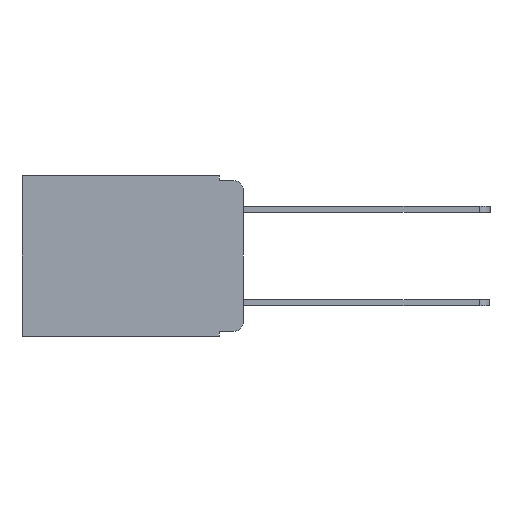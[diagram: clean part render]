
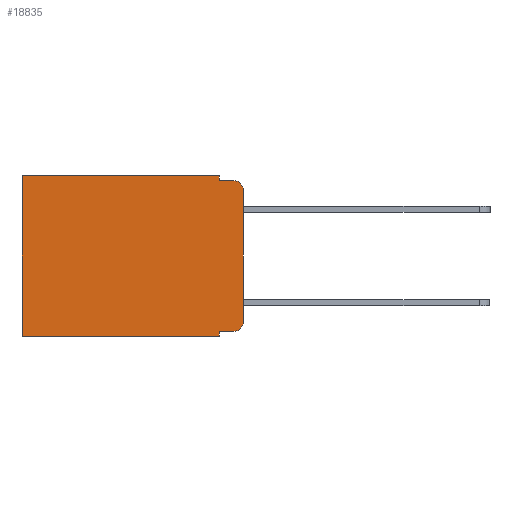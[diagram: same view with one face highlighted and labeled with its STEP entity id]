
A CAD part, left-side view. The second image highlights one B-rep face of the part: STEP entity #18835.
In plain terms, the highlighted planar face has unit normal (-1, 0, 0).
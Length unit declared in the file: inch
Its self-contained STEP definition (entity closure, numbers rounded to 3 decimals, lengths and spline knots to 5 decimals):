
#89 = VERTEX_POINT ( 'NONE', #7108 ) ;
#629 = ORIENTED_EDGE ( 'NONE', *, *, #4387, .T. ) ;
#857 = VERTEX_POINT ( 'NONE', #22452 ) ;
#1180 = FACE_OUTER_BOUND ( 'NONE', #19927, .T. ) ;
#1786 = CARTESIAN_POINT ( 'NONE',  ( 0.298, 0.051, -0.343 ) ) ;
#1888 = CARTESIAN_POINT ( 'NONE',  ( 0.298, 0.02, -0.03 ) ) ;
#2769 = CARTESIAN_POINT ( 'NONE',  ( 0.298, 0., 0. ) ) ;
#2882 = CARTESIAN_POINT ( 'NONE',  ( 0.298, 0., -0.03 ) ) ;
#2957 = CARTESIAN_POINT ( 'NONE',  ( 0.298, 0.051, -0.01 ) ) ;
#3041 = VERTEX_POINT ( 'NONE', #2882 ) ;
#3230 = VERTEX_POINT ( 'NONE', #14406 ) ;
#3738 = DIRECTION ( 'NONE',  ( 0., 0., -1. ) ) ;
#4284 = LINE ( 'NONE', #2769, #21764 ) ;
#4387 = EDGE_CURVE ( 'NONE', #3041, #89, #19118, .T. ) ;
#4490 = EDGE_CURVE ( 'NONE', #5047, #8650, #21510, .T. ) ;
#4580 = VERTEX_POINT ( 'NONE', #14867 ) ;
#4734 = EDGE_CURVE ( 'NONE', #3041, #9406, #4284, .T. ) ;
#4835 = CARTESIAN_POINT ( 'NONE',  ( 0.298, 0.051, -0.333 ) ) ;
#5047 = VERTEX_POINT ( 'NONE', #1786 ) ;
#5217 = AXIS2_PLACEMENT_3D ( 'NONE', #8391, #20550, #10196 ) ;
#5502 = EDGE_CURVE ( 'NONE', #4580, #18981, #6504, .T. ) ;
#5528 = VECTOR ( 'NONE', #20589, 39.37008 ) ;
#5563 = LINE ( 'NONE', #18065, #11428 ) ;
#5821 = DIRECTION ( 'NONE',  ( 0., 0., -1. ) ) ;
#6057 = CARTESIAN_POINT ( 'NONE',  ( 0.298, 0., 0. ) ) ;
#6140 = DIRECTION ( 'NONE',  ( 0., 0., -1. ) ) ;
#6504 = LINE ( 'NONE', #6858, #19861 ) ;
#6658 = ORIENTED_EDGE ( 'NONE', *, *, #5502, .F. ) ;
#6824 = CARTESIAN_POINT ( 'NONE',  ( 0.298, 0., -0.313 ) ) ;
#6858 = CARTESIAN_POINT ( 'NONE',  ( 0.298, 0.051, 0. ) ) ;
#7108 = CARTESIAN_POINT ( 'NONE',  ( 0.298, 0.02, -0.01 ) ) ;
#7143 = DIRECTION ( 'NONE',  ( 0., 1., 0. ) ) ;
#7154 = EDGE_CURVE ( 'NONE', #12193, #8650, #5563, .T. ) ;
#7475 = EDGE_CURVE ( 'NONE', #4580, #12193, #20570, .T. ) ;
#7652 = VECTOR ( 'NONE', #21484, 39.37008 ) ;
#7845 = DIRECTION ( 'NONE',  ( 1., 0., 0. ) ) ;
#7990 = EDGE_CURVE ( 'NONE', #18981, #89, #19481, .T. ) ;
#8359 = ORIENTED_EDGE ( 'NONE', *, *, #17285, .T. ) ;
#8391 = CARTESIAN_POINT ( 'NONE',  ( 0.298, 0.02, -0.313 ) ) ;
#8650 = VERTEX_POINT ( 'NONE', #13787 ) ;
#9406 = VERTEX_POINT ( 'NONE', #6824 ) ;
#9649 = VECTOR ( 'NONE', #6140, 39.37008 ) ;
#10167 = AXIS2_PLACEMENT_3D ( 'NONE', #6057, #7845, #20012 ) ;
#10196 = DIRECTION ( 'NONE',  ( 0., 0., -1. ) ) ;
#10237 = CARTESIAN_POINT ( 'NONE',  ( 0.298, 0.051, -0.01 ) ) ;
#10572 = ORIENTED_EDGE ( 'NONE', *, *, #4490, .F. ) ;
#11428 = VECTOR ( 'NONE', #5821, 39.37008 ) ;
#11933 = EDGE_CURVE ( 'NONE', #3230, #857, #18338, .T. ) ;
#11976 = VECTOR ( 'NONE', #7143, 39.37008 ) ;
#12193 = VERTEX_POINT ( 'NONE', #17762 ) ;
#13209 = CARTESIAN_POINT ( 'NONE',  ( 0.298, 0.051, 0. ) ) ;
#13787 = CARTESIAN_POINT ( 'NONE',  ( 0.298, 0.473, -0.343 ) ) ;
#13816 = VECTOR ( 'NONE', #18933, 39.37008 ) ;
#13884 = ORIENTED_EDGE ( 'NONE', *, *, #7990, .F. ) ;
#14167 = ORIENTED_EDGE ( 'NONE', *, *, #18858, .F. ) ;
#14359 = LINE ( 'NONE', #13209, #9649 ) ;
#14406 = CARTESIAN_POINT ( 'NONE',  ( 0.298, 0.051, -0.333 ) ) ;
#14413 = DIRECTION ( 'NONE',  ( -1., 0., 0. ) ) ;
#14867 = CARTESIAN_POINT ( 'NONE',  ( 0.298, 0.051, 0. ) ) ;
#15244 = DIRECTION ( 'NONE',  ( 0., 0., -1. ) ) ;
#16026 = ORIENTED_EDGE ( 'NONE', *, *, #7154, .T. ) ;
#16262 = CARTESIAN_POINT ( 'NONE',  ( 0.298, 0., -0.343 ) ) ;
#16579 = PLANE ( 'NONE',  #10167 ) ;
#17285 = EDGE_CURVE ( 'NONE', #857, #9406, #22663, .T. ) ;
#17301 = ORIENTED_EDGE ( 'NONE', *, *, #4734, .F. ) ;
#17587 = CARTESIAN_POINT ( 'NONE',  ( 0.298, 0., 0. ) ) ;
#17762 = CARTESIAN_POINT ( 'NONE',  ( 0.298, 0.473, 0. ) ) ;
#18065 = CARTESIAN_POINT ( 'NONE',  ( 0.298, 0.473, 0. ) ) ;
#18338 = LINE ( 'NONE', #4835, #13816 ) ;
#18835 = ADVANCED_FACE ( 'NONE', ( #1180 ), #16579, .F. ) ;
#18858 = EDGE_CURVE ( 'NONE', #3230, #5047, #14359, .T. ) ;
#18933 = DIRECTION ( 'NONE',  ( 0., -1., 0. ) ) ;
#18981 = VERTEX_POINT ( 'NONE', #2957 ) ;
#19118 = CIRCLE ( 'NONE', #21300, 0.02 ) ;
#19481 = LINE ( 'NONE', #10237, #5528 ) ;
#19861 = VECTOR ( 'NONE', #22450, 39.37008 ) ;
#19927 = EDGE_LOOP ( 'NONE', ( #17301, #629, #13884, #6658, #22158, #16026, #10572, #14167, #20321, #8359 ) ) ;
#20012 = DIRECTION ( 'NONE',  ( 0., 0., -1. ) ) ;
#20321 = ORIENTED_EDGE ( 'NONE', *, *, #11933, .T. ) ;
#20550 = DIRECTION ( 'NONE',  ( -1., 0., 0. ) ) ;
#20570 = LINE ( 'NONE', #17587, #11976 ) ;
#20589 = DIRECTION ( 'NONE',  ( 0., -1., 0. ) ) ;
#21300 = AXIS2_PLACEMENT_3D ( 'NONE', #1888, #14413, #3738 ) ;
#21484 = DIRECTION ( 'NONE',  ( 0., 1., 0. ) ) ;
#21510 = LINE ( 'NONE', #16262, #7652 ) ;
#21764 = VECTOR ( 'NONE', #15244, 39.37008 ) ;
#22158 = ORIENTED_EDGE ( 'NONE', *, *, #7475, .T. ) ;
#22450 = DIRECTION ( 'NONE',  ( 0., 0., -1. ) ) ;
#22452 = CARTESIAN_POINT ( 'NONE',  ( 0.298, 0.02, -0.333 ) ) ;
#22663 = CIRCLE ( 'NONE', #5217, 0.02 ) ;
